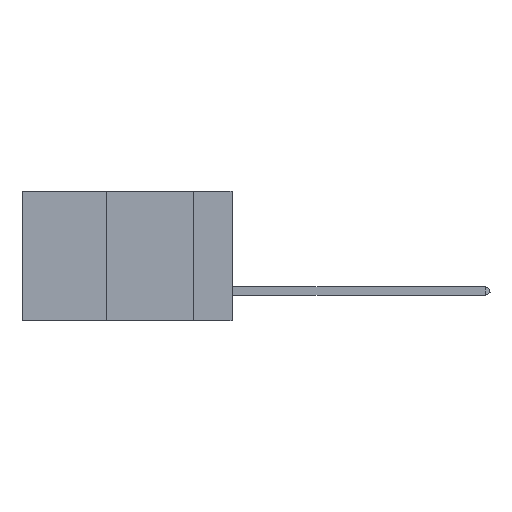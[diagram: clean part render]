
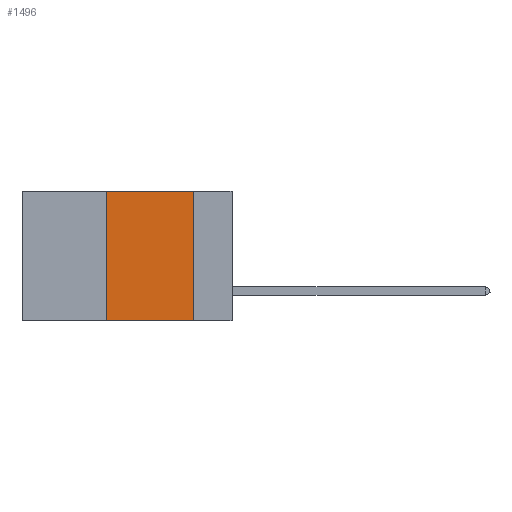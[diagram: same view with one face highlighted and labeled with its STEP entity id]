
A CAD part, left-side view. The second image highlights one B-rep face of the part: STEP entity #1496.
In plain terms, the highlighted planar face has unit normal (-1, 0, 0).
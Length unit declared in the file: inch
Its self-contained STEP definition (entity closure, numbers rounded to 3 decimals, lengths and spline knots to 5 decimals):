
#142 = CARTESIAN_POINT ( 'NONE',  ( 0., 0.11, 0. ) ) ;
#928 = VECTOR ( 'NONE', #7350, 39.37008 ) ;
#1027 = FACE_OUTER_BOUND ( 'NONE', #1172, .T. ) ;
#1136 = CARTESIAN_POINT ( 'NONE',  ( 0., 0.6, 0. ) ) ;
#1172 = EDGE_LOOP ( 'NONE', ( #2526, #7040, #13407, #2443 ) ) ;
#1496 = ADVANCED_FACE ( 'NONE', ( #1027 ), #7076, .F. ) ;
#1662 = DIRECTION ( 'NONE',  ( 0., 0., -1. ) ) ;
#1751 = DIRECTION ( 'NONE',  ( 0., 0., 1. ) ) ;
#2443 = ORIENTED_EDGE ( 'NONE', *, *, #2499, .T. ) ;
#2499 = EDGE_CURVE ( 'NONE', #12690, #6983, #12890, .T. ) ;
#2526 = ORIENTED_EDGE ( 'NONE', *, *, #5377, .F. ) ;
#2840 = VERTEX_POINT ( 'NONE', #142 ) ;
#3312 = LINE ( 'NONE', #5581, #8604 ) ;
#3684 = CARTESIAN_POINT ( 'NONE',  ( 0., 0.36, -0.37 ) ) ;
#5190 = DIRECTION ( 'NONE',  ( 0., -1., 0. ) ) ;
#5297 = EDGE_CURVE ( 'NONE', #12690, #10364, #14383, .T. ) ;
#5377 = EDGE_CURVE ( 'NONE', #2840, #6983, #3312, .T. ) ;
#5581 = CARTESIAN_POINT ( 'NONE',  ( 0., 0.11, 0. ) ) ;
#5899 = DIRECTION ( 'NONE',  ( 0., 0., -1. ) ) ;
#6157 = VECTOR ( 'NONE', #5190, 39.37008 ) ;
#6983 = VERTEX_POINT ( 'NONE', #8012 ) ;
#7021 = CARTESIAN_POINT ( 'NONE',  ( 0., 0.6, 0. ) ) ;
#7040 = ORIENTED_EDGE ( 'NONE', *, *, #15154, .F. ) ;
#7076 = PLANE ( 'NONE',  #13933 ) ;
#7350 = DIRECTION ( 'NONE',  ( 0., -1., 0. ) ) ;
#8001 = CARTESIAN_POINT ( 'NONE',  ( 0., 0.36, 0. ) ) ;
#8012 = CARTESIAN_POINT ( 'NONE',  ( 0., 0.11, -0.37 ) ) ;
#8604 = VECTOR ( 'NONE', #1662, 39.37008 ) ;
#9896 = CARTESIAN_POINT ( 'NONE',  ( 0., 0.36, 0. ) ) ;
#10364 = VERTEX_POINT ( 'NONE', #9896 ) ;
#11493 = CARTESIAN_POINT ( 'NONE',  ( 0., 0.6, -0.37 ) ) ;
#11977 = VECTOR ( 'NONE', #1751, 39.37008 ) ;
#12095 = DIRECTION ( 'NONE',  ( 1., 0., 0. ) ) ;
#12690 = VERTEX_POINT ( 'NONE', #3684 ) ;
#12890 = LINE ( 'NONE', #11493, #6157 ) ;
#13407 = ORIENTED_EDGE ( 'NONE', *, *, #5297, .F. ) ;
#13933 = AXIS2_PLACEMENT_3D ( 'NONE', #7021, #12095, #5899 ) ;
#13945 = LINE ( 'NONE', #1136, #928 ) ;
#14383 = LINE ( 'NONE', #8001, #11977 ) ;
#15154 = EDGE_CURVE ( 'NONE', #10364, #2840, #13945, .T. ) ;
